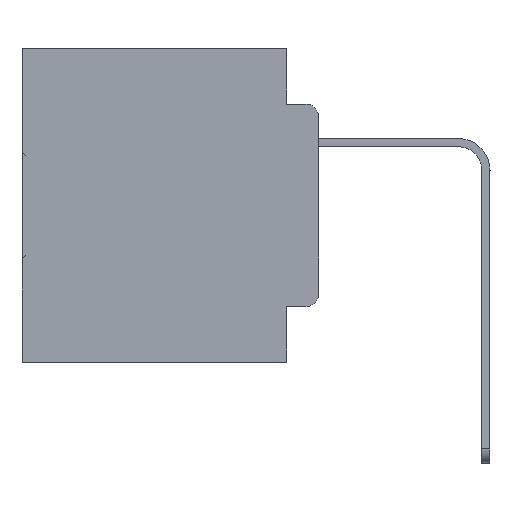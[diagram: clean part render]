
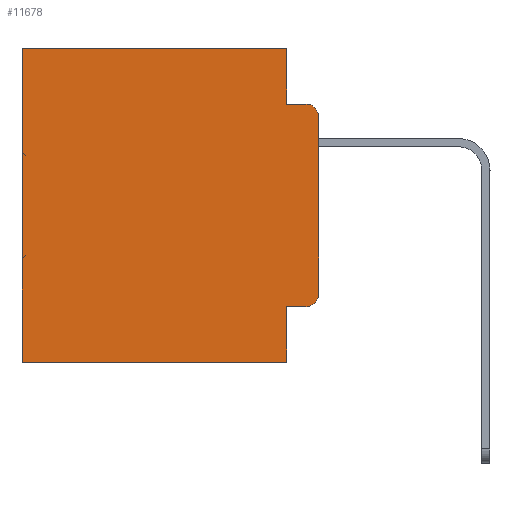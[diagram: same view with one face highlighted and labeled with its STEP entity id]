
A CAD part, left-side view. The second image highlights one B-rep face of the part: STEP entity #11678.
In plain terms, the highlighted planar face has unit normal (-1, 0, 0).
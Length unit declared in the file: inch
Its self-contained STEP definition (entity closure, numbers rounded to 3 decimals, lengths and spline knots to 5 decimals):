
#143 = EDGE_CURVE ( 'NONE', #21220, #31382, #3537, .T. ) ;
#609 = DIRECTION ( 'NONE',  ( -1., 0., 0. ) ) ;
#975 = CARTESIAN_POINT ( 'NONE',  ( 0.298, 0.051, 0. ) ) ;
#1405 = ORIENTED_EDGE ( 'NONE', *, *, #143, .T. ) ;
#1426 = FACE_OUTER_BOUND ( 'NONE', #11416, .T. ) ;
#2326 = CIRCLE ( 'NONE', #22518, 0.02 ) ;
#2627 = VERTEX_POINT ( 'NONE', #15343 ) ;
#3537 = LINE ( 'NONE', #27449, #18229 ) ;
#4278 = LINE ( 'NONE', #975, #21384 ) ;
#4744 = DIRECTION ( 'NONE',  ( -1., 0., 0. ) ) ;
#6519 = EDGE_CURVE ( 'NONE', #14046, #7103, #2326, .T. ) ;
#6531 = ORIENTED_EDGE ( 'NONE', *, *, #30768, .F. ) ;
#6553 = CARTESIAN_POINT ( 'NONE',  ( 0.298, 0., -0.5 ) ) ;
#7090 = VECTOR ( 'NONE', #10246, 39.37008 ) ;
#7103 = VERTEX_POINT ( 'NONE', #16530 ) ;
#7259 = ORIENTED_EDGE ( 'NONE', *, *, #31480, .T. ) ;
#7372 = LINE ( 'NONE', #32714, #28471 ) ;
#7530 = VERTEX_POINT ( 'NONE', #23656 ) ;
#7583 = VERTEX_POINT ( 'NONE', #26087 ) ;
#7800 = LINE ( 'NONE', #32756, #26518 ) ;
#8567 = CARTESIAN_POINT ( 'NONE',  ( 0.298, 0.051, -0.0885 ) ) ;
#8930 = AXIS2_PLACEMENT_3D ( 'NONE', #14441, #12206, #22684 ) ;
#8982 = EDGE_CURVE ( 'NONE', #31382, #7583, #19450, .T. ) ;
#9727 = AXIS2_PLACEMENT_3D ( 'NONE', #20072, #4744, #27325 ) ;
#9911 = VECTOR ( 'NONE', #15702, 39.37008 ) ;
#10039 = CARTESIAN_POINT ( 'NONE',  ( 0.298, 0.051, -0.5 ) ) ;
#10246 = DIRECTION ( 'NONE',  ( 0., 0., -1. ) ) ;
#11193 = CARTESIAN_POINT ( 'NONE',  ( 0.298, 0.051, -0.4115 ) ) ;
#11416 = EDGE_LOOP ( 'NONE', ( #18779, #32503, #17843, #17648, #1405, #18576, #6531, #28809, #27180, #7259 ) ) ;
#11678 = ADVANCED_FACE ( 'NONE', ( #1426 ), #21920, .F. ) ;
#12193 = DIRECTION ( 'NONE',  ( 0., 1., 0. ) ) ;
#12206 = DIRECTION ( 'NONE',  ( 1., 0., 0. ) ) ;
#12242 = VECTOR ( 'NONE', #28190, 39.37008 ) ;
#12619 = CARTESIAN_POINT ( 'NONE',  ( 0.298, 0., 0. ) ) ;
#14046 = VERTEX_POINT ( 'NONE', #19941 ) ;
#14122 = EDGE_CURVE ( 'NONE', #24690, #7530, #7372, .T. ) ;
#14441 = CARTESIAN_POINT ( 'NONE',  ( 0.298, 0., 0. ) ) ;
#15343 = CARTESIAN_POINT ( 'NONE',  ( 0.298, 0., -0.3915 ) ) ;
#15702 = DIRECTION ( 'NONE',  ( 0., 0., -1. ) ) ;
#16530 = CARTESIAN_POINT ( 'NONE',  ( 0.298, 0.02, -0.0885 ) ) ;
#16755 = LINE ( 'NONE', #6553, #27119 ) ;
#17648 = ORIENTED_EDGE ( 'NONE', *, *, #18759, .F. ) ;
#17724 = CARTESIAN_POINT ( 'NONE',  ( 0.298, 0.473, 0. ) ) ;
#17843 = ORIENTED_EDGE ( 'NONE', *, *, #19880, .F. ) ;
#18229 = VECTOR ( 'NONE', #12193, 39.37008 ) ;
#18487 = CARTESIAN_POINT ( 'NONE',  ( 0.298, 0.051, 0. ) ) ;
#18576 = ORIENTED_EDGE ( 'NONE', *, *, #8982, .T. ) ;
#18598 = VERTEX_POINT ( 'NONE', #10039 ) ;
#18759 = EDGE_CURVE ( 'NONE', #21220, #23252, #4278, .T. ) ;
#18779 = ORIENTED_EDGE ( 'NONE', *, *, #22332, .F. ) ;
#19450 = LINE ( 'NONE', #17724, #7090 ) ;
#19843 = DIRECTION ( 'NONE',  ( 0., -1., 0. ) ) ;
#19880 = EDGE_CURVE ( 'NONE', #23252, #7103, #7800, .T. ) ;
#19941 = CARTESIAN_POINT ( 'NONE',  ( 0.298, 0., -0.1085 ) ) ;
#20072 = CARTESIAN_POINT ( 'NONE',  ( 0.298, 0.02, -0.3915 ) ) ;
#20935 = DIRECTION ( 'NONE',  ( 0., 0., -1. ) ) ;
#21220 = VERTEX_POINT ( 'NONE', #18487 ) ;
#21384 = VECTOR ( 'NONE', #26175, 39.37008 ) ;
#21920 = PLANE ( 'NONE',  #8930 ) ;
#22332 = EDGE_CURVE ( 'NONE', #14046, #2627, #25786, .T. ) ;
#22518 = AXIS2_PLACEMENT_3D ( 'NONE', #28585, #609, #20935 ) ;
#22684 = DIRECTION ( 'NONE',  ( 0., 0., -1. ) ) ;
#23115 = DIRECTION ( 'NONE',  ( 0., -1., 0. ) ) ;
#23252 = VERTEX_POINT ( 'NONE', #8567 ) ;
#23656 = CARTESIAN_POINT ( 'NONE',  ( 0.298, 0.02, -0.4115 ) ) ;
#24325 = CARTESIAN_POINT ( 'NONE',  ( 0.298, 0.473, 0. ) ) ;
#24690 = VERTEX_POINT ( 'NONE', #11193 ) ;
#25786 = LINE ( 'NONE', #12619, #12242 ) ;
#26087 = CARTESIAN_POINT ( 'NONE',  ( 0.298, 0.473, -0.5 ) ) ;
#26175 = DIRECTION ( 'NONE',  ( 0., 0., -1. ) ) ;
#26518 = VECTOR ( 'NONE', #23115, 39.37008 ) ;
#26587 = DIRECTION ( 'NONE',  ( 0., 1., 0. ) ) ;
#27119 = VECTOR ( 'NONE', #26587, 39.37008 ) ;
#27180 = ORIENTED_EDGE ( 'NONE', *, *, #14122, .T. ) ;
#27325 = DIRECTION ( 'NONE',  ( 0., 0., -1. ) ) ;
#27449 = CARTESIAN_POINT ( 'NONE',  ( 0.298, 0., 0. ) ) ;
#27838 = CIRCLE ( 'NONE', #9727, 0.02 ) ;
#28190 = DIRECTION ( 'NONE',  ( 0., 0., -1. ) ) ;
#28471 = VECTOR ( 'NONE', #19843, 39.37008 ) ;
#28585 = CARTESIAN_POINT ( 'NONE',  ( 0.298, 0.02, -0.1085 ) ) ;
#28809 = ORIENTED_EDGE ( 'NONE', *, *, #32295, .F. ) ;
#30205 = LINE ( 'NONE', #30910, #9911 ) ;
#30768 = EDGE_CURVE ( 'NONE', #18598, #7583, #16755, .T. ) ;
#30910 = CARTESIAN_POINT ( 'NONE',  ( 0.298, 0.051, 0. ) ) ;
#31382 = VERTEX_POINT ( 'NONE', #24325 ) ;
#31480 = EDGE_CURVE ( 'NONE', #7530, #2627, #27838, .T. ) ;
#32295 = EDGE_CURVE ( 'NONE', #24690, #18598, #30205, .T. ) ;
#32503 = ORIENTED_EDGE ( 'NONE', *, *, #6519, .T. ) ;
#32714 = CARTESIAN_POINT ( 'NONE',  ( 0.298, 0.051, -0.4115 ) ) ;
#32756 = CARTESIAN_POINT ( 'NONE',  ( 0.298, 0.051, -0.0885 ) ) ;
